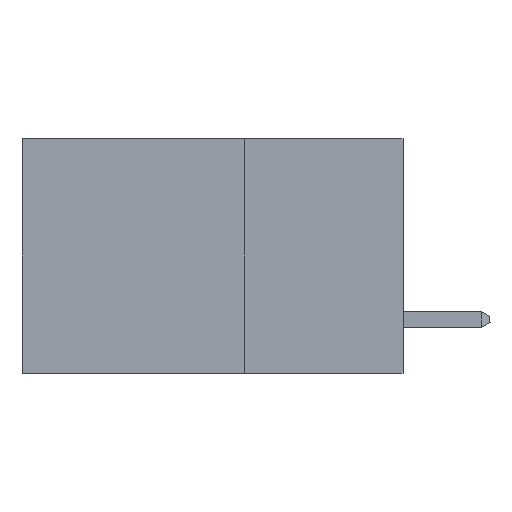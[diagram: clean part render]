
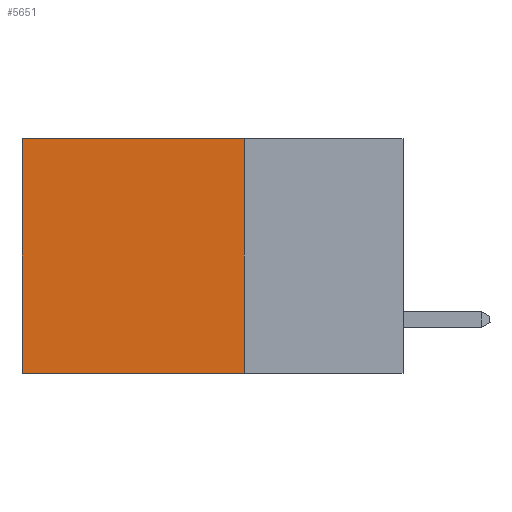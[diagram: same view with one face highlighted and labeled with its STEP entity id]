
A CAD part, left-side view. The second image highlights one B-rep face of the part: STEP entity #5651.
In plain terms, the highlighted planar face has unit normal (-1, 0, 0).
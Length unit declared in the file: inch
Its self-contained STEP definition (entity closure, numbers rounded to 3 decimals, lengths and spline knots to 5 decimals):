
#1569 = VERTEX_POINT ( 'NONE', #13316 ) ;
#1652 = EDGE_CURVE ( 'NONE', #21084, #1569, #14410, .T. ) ;
#2314 = CARTESIAN_POINT ( 'NONE',  ( 0.2875, 0.25, 0. ) ) ;
#4632 = CARTESIAN_POINT ( 'NONE',  ( 0.2875, 0.25, -0.37 ) ) ;
#5128 = DIRECTION ( 'NONE',  ( 0., 0., -1. ) ) ;
#5523 = DIRECTION ( 'NONE',  ( 0., 1., 0. ) ) ;
#5651 = ADVANCED_FACE ( 'NONE', ( #15983 ), #21820, .F. ) ;
#6751 = CARTESIAN_POINT ( 'NONE',  ( 0.2875, 0.6, 0. ) ) ;
#6971 = EDGE_CURVE ( 'NONE', #7903, #1569, #10027, .T. ) ;
#7903 = VERTEX_POINT ( 'NONE', #14240 ) ;
#10027 = LINE ( 'NONE', #6751, #21106 ) ;
#10712 = VECTOR ( 'NONE', #22082, 39.37008 ) ;
#11452 = DIRECTION ( 'NONE',  ( 0., 1., 0. ) ) ;
#11927 = EDGE_CURVE ( 'NONE', #25661, #21084, #25927, .T. ) ;
#12327 = VECTOR ( 'NONE', #11452, 39.37008 ) ;
#13316 = CARTESIAN_POINT ( 'NONE',  ( 0.2875, 0.6, -0.37 ) ) ;
#14240 = CARTESIAN_POINT ( 'NONE',  ( 0.2875, 0.6, 0. ) ) ;
#14410 = LINE ( 'NONE', #4632, #12327 ) ;
#15263 = DIRECTION ( 'NONE',  ( 1., 0., 0. ) ) ;
#15347 = DIRECTION ( 'NONE',  ( 0., 0., -1. ) ) ;
#15825 = ORIENTED_EDGE ( 'NONE', *, *, #11927, .F. ) ;
#15983 = FACE_OUTER_BOUND ( 'NONE', #26754, .T. ) ;
#16742 = ORIENTED_EDGE ( 'NONE', *, *, #1652, .F. ) ;
#21084 = VERTEX_POINT ( 'NONE', #26160 ) ;
#21092 = ORIENTED_EDGE ( 'NONE', *, *, #24476, .T. ) ;
#21106 = VECTOR ( 'NONE', #5128, 39.37008 ) ;
#21330 = AXIS2_PLACEMENT_3D ( 'NONE', #23956, #15263, #15347 ) ;
#21820 = PLANE ( 'NONE',  #21330 ) ;
#22082 = DIRECTION ( 'NONE',  ( 0., 0., -1. ) ) ;
#23956 = CARTESIAN_POINT ( 'NONE',  ( 0.2875, 0.25, 0. ) ) ;
#24476 = EDGE_CURVE ( 'NONE', #25661, #7903, #28430, .T. ) ;
#24983 = VECTOR ( 'NONE', #5523, 39.37008 ) ;
#25312 = CARTESIAN_POINT ( 'NONE',  ( 0.2875, 0.25, 0. ) ) ;
#25661 = VERTEX_POINT ( 'NONE', #28107 ) ;
#25927 = LINE ( 'NONE', #2314, #10712 ) ;
#26123 = ORIENTED_EDGE ( 'NONE', *, *, #6971, .T. ) ;
#26160 = CARTESIAN_POINT ( 'NONE',  ( 0.2875, 0.25, -0.37 ) ) ;
#26754 = EDGE_LOOP ( 'NONE', ( #26123, #16742, #15825, #21092 ) ) ;
#28107 = CARTESIAN_POINT ( 'NONE',  ( 0.2875, 0.25, 0. ) ) ;
#28430 = LINE ( 'NONE', #25312, #24983 ) ;
